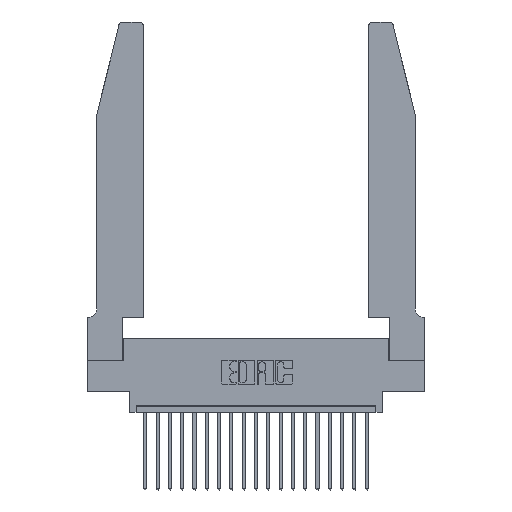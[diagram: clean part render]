
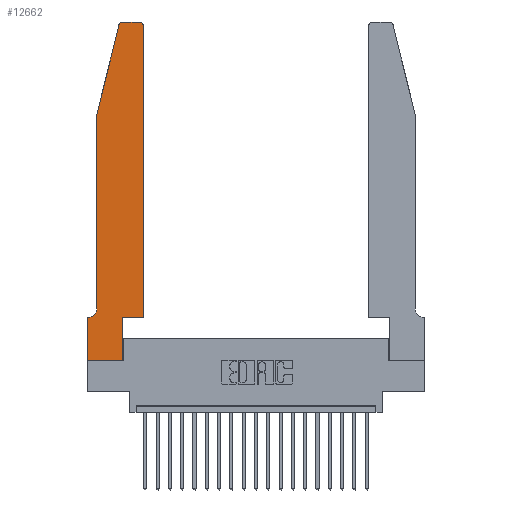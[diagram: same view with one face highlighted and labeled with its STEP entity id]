
A CAD part, top view. The second image highlights one B-rep face of the part: STEP entity #12662.
In plain terms, the highlighted planar face has unit normal (0, 0, 1).
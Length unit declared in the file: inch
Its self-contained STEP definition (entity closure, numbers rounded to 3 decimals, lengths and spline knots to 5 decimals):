
#102 = VECTOR ( 'NONE', #16913, 39.37008 ) ;
#257 = DIRECTION ( 'NONE',  ( 0., 0., -1. ) ) ;
#327 = CARTESIAN_POINT ( 'NONE',  ( 0.284, 2.75, 0.37 ) ) ;
#587 = AXIS2_PLACEMENT_3D ( 'NONE', #10549, #257, #5516 ) ;
#880 = ORIENTED_EDGE ( 'NONE', *, *, #9797, .T. ) ;
#1093 = VERTEX_POINT ( 'NONE', #22178 ) ;
#1176 = LINE ( 'NONE', #9467, #5963 ) ;
#1204 = VECTOR ( 'NONE', #10501, 39.37008 ) ;
#1364 = EDGE_CURVE ( 'NONE', #2460, #10836, #12725, .T. ) ;
#1492 = DIRECTION ( 'NONE',  ( -1., 0., 0. ) ) ;
#1579 = DIRECTION ( 'NONE',  ( 0., 0., 1. ) ) ;
#1655 = DIRECTION ( 'NONE',  ( 1., 0., 0. ) ) ;
#2086 = EDGE_LOOP ( 'NONE', ( #8079, #880, #11251, #3772, #17638, #19984, #12000, #12887, #15608, #21807, #15028, #2759 ) ) ;
#2460 = VERTEX_POINT ( 'NONE', #17323 ) ;
#2746 = LINE ( 'NONE', #17678, #9189 ) ;
#2759 = ORIENTED_EDGE ( 'NONE', *, *, #18175, .T. ) ;
#3187 = VERTEX_POINT ( 'NONE', #327 ) ;
#3426 = EDGE_CURVE ( 'NONE', #8531, #3187, #22290, .T. ) ;
#3436 = LINE ( 'NONE', #16147, #5274 ) ;
#3772 = ORIENTED_EDGE ( 'NONE', *, *, #13375, .T. ) ;
#3917 = CARTESIAN_POINT ( 'NONE',  ( 0.0755, 2., 0.37 ) ) ;
#4987 = VECTOR ( 'NONE', #1492, 39.37008 ) ;
#5092 = VECTOR ( 'NONE', #13728, 39.37008 ) ;
#5165 = LINE ( 'NONE', #13865, #1204 ) ;
#5274 = VECTOR ( 'NONE', #7617, 39.37008 ) ;
#5516 = DIRECTION ( 'NONE',  ( -1., 0., 0. ) ) ;
#5618 = CARTESIAN_POINT ( 'NONE',  ( 0.0755, 0.35, 0.37 ) ) ;
#5963 = VECTOR ( 'NONE', #7849, 39.37008 ) ;
#6348 = CARTESIAN_POINT ( 'NONE',  ( 0.4505, 0.35, 0.37 ) ) ;
#6683 = EDGE_CURVE ( 'NONE', #11929, #21466, #3436, .T. ) ;
#7617 = DIRECTION ( 'NONE',  ( 0., 1., 0. ) ) ;
#7849 = DIRECTION ( 'NONE',  ( -0.239, -0.971, 0. ) ) ;
#8027 = LINE ( 'NONE', #12352, #20471 ) ;
#8079 = ORIENTED_EDGE ( 'NONE', *, *, #3426, .T. ) ;
#8176 = CARTESIAN_POINT ( 'NONE',  ( 0.4505, 2.72, 0.37 ) ) ;
#8531 = VERTEX_POINT ( 'NONE', #11025 ) ;
#9189 = VECTOR ( 'NONE', #16290, 39.37008 ) ;
#9215 = DIRECTION ( 'NONE',  ( -1., 0., 0. ) ) ;
#9467 = CARTESIAN_POINT ( 'NONE',  ( 0.0755, 2., 0.37 ) ) ;
#9570 = EDGE_CURVE ( 'NONE', #10180, #21219, #1176, .T. ) ;
#9797 = EDGE_CURVE ( 'NONE', #3187, #10180, #21102, .T. ) ;
#9818 = CARTESIAN_POINT ( 'NONE',  ( 0.284, 2.72, 0.37 ) ) ;
#9907 = CARTESIAN_POINT ( 'NONE',  ( 0.2865, 0.35, 0.37 ) ) ;
#10023 = DIRECTION ( 'NONE',  ( 1., 0., 0. ) ) ;
#10119 = CARTESIAN_POINT ( 'NONE',  ( 0., 0.35, 0.37 ) ) ;
#10157 = VECTOR ( 'NONE', #9215, 39.37008 ) ;
#10180 = VERTEX_POINT ( 'NONE', #12488 ) ;
#10501 = DIRECTION ( 'NONE',  ( 0., -1., 0. ) ) ;
#10549 = CARTESIAN_POINT ( 'NONE',  ( 0.0055, 0.42, 0.37 ) ) ;
#10703 = EDGE_CURVE ( 'NONE', #12597, #15881, #11671, .T. ) ;
#10836 = VERTEX_POINT ( 'NONE', #12690 ) ;
#10906 = VERTEX_POINT ( 'NONE', #9907 ) ;
#11025 = CARTESIAN_POINT ( 'NONE',  ( 0.4205, 2.75, 0.37 ) ) ;
#11251 = ORIENTED_EDGE ( 'NONE', *, *, #9570, .T. ) ;
#11536 = LINE ( 'NONE', #5618, #10157 ) ;
#11671 = CIRCLE ( 'NONE', #587, 0.07 ) ;
#11929 = VERTEX_POINT ( 'NONE', #12266 ) ;
#11979 = PLANE ( 'NONE',  #20167 ) ;
#12000 = ORIENTED_EDGE ( 'NONE', *, *, #15579, .T. ) ;
#12266 = CARTESIAN_POINT ( 'NONE',  ( 0.4505, 0.35, 0.37 ) ) ;
#12352 = CARTESIAN_POINT ( 'NONE',  ( 0., 0., 0.37 ) ) ;
#12488 = CARTESIAN_POINT ( 'NONE',  ( 0.25487, 2.72718, 0.37 ) ) ;
#12597 = VERTEX_POINT ( 'NONE', #18252 ) ;
#12662 = ADVANCED_FACE ( 'NONE', ( #21810 ), #11979, .T. ) ;
#12690 = CARTESIAN_POINT ( 'NONE',  ( 0.2865, 0., 0.37 ) ) ;
#12725 = LINE ( 'NONE', #22132, #5092 ) ;
#12872 = CIRCLE ( 'NONE', #14755, 0.03 ) ;
#12887 = ORIENTED_EDGE ( 'NONE', *, *, #1364, .T. ) ;
#13375 = EDGE_CURVE ( 'NONE', #21219, #12597, #5165, .T. ) ;
#13404 = EDGE_CURVE ( 'NONE', #10906, #11929, #14656, .T. ) ;
#13728 = DIRECTION ( 'NONE',  ( 1., 0., 0. ) ) ;
#13865 = CARTESIAN_POINT ( 'NONE',  ( 0.0755, 2., 0.37 ) ) ;
#14656 = LINE ( 'NONE', #6348, #102 ) ;
#14755 = AXIS2_PLACEMENT_3D ( 'NONE', #18395, #22085, #10023 ) ;
#14777 = EDGE_CURVE ( 'NONE', #10836, #10906, #2746, .T. ) ;
#15028 = ORIENTED_EDGE ( 'NONE', *, *, #6683, .T. ) ;
#15579 = EDGE_CURVE ( 'NONE', #1093, #2460, #8027, .T. ) ;
#15608 = ORIENTED_EDGE ( 'NONE', *, *, #14777, .T. ) ;
#15784 = DIRECTION ( 'NONE',  ( 0., -1., 0. ) ) ;
#15881 = VERTEX_POINT ( 'NONE', #17670 ) ;
#16147 = CARTESIAN_POINT ( 'NONE',  ( 0.4505, 0.35, 0.37 ) ) ;
#16290 = DIRECTION ( 'NONE',  ( 0., 1., 0. ) ) ;
#16913 = DIRECTION ( 'NONE',  ( 1., 0., 0. ) ) ;
#17323 = CARTESIAN_POINT ( 'NONE',  ( 0., 0., 0.37 ) ) ;
#17638 = ORIENTED_EDGE ( 'NONE', *, *, #10703, .T. ) ;
#17670 = CARTESIAN_POINT ( 'NONE',  ( 0.0055, 0.35, 0.37 ) ) ;
#17678 = CARTESIAN_POINT ( 'NONE',  ( 0.2865, 0.35, 0.37 ) ) ;
#17866 = EDGE_CURVE ( 'NONE', #15881, #1093, #11536, .T. ) ;
#18175 = EDGE_CURVE ( 'NONE', #21466, #8531, #12872, .T. ) ;
#18252 = CARTESIAN_POINT ( 'NONE',  ( 0.0755, 0.42, 0.37 ) ) ;
#18395 = CARTESIAN_POINT ( 'NONE',  ( 0.4205, 2.72, 0.37 ) ) ;
#19984 = ORIENTED_EDGE ( 'NONE', *, *, #17866, .T. ) ;
#20167 = AXIS2_PLACEMENT_3D ( 'NONE', #10119, #1579, #1655 ) ;
#20438 = CARTESIAN_POINT ( 'NONE',  ( 0.2605, 2.75, 0.37 ) ) ;
#20471 = VECTOR ( 'NONE', #15784, 39.37008 ) ;
#20517 = DIRECTION ( 'NONE',  ( 1., 0., 0. ) ) ;
#21102 = CIRCLE ( 'NONE', #21491, 0.03 ) ;
#21219 = VERTEX_POINT ( 'NONE', #3917 ) ;
#21466 = VERTEX_POINT ( 'NONE', #8176 ) ;
#21491 = AXIS2_PLACEMENT_3D ( 'NONE', #9818, #21879, #20517 ) ;
#21807 = ORIENTED_EDGE ( 'NONE', *, *, #13404, .T. ) ;
#21810 = FACE_OUTER_BOUND ( 'NONE', #2086, .T. ) ;
#21879 = DIRECTION ( 'NONE',  ( 0., 0., 1. ) ) ;
#22085 = DIRECTION ( 'NONE',  ( 0., 0., 1. ) ) ;
#22132 = CARTESIAN_POINT ( 'NONE',  ( 0., 0., 0.37 ) ) ;
#22178 = CARTESIAN_POINT ( 'NONE',  ( 0., 0.35, 0.37 ) ) ;
#22290 = LINE ( 'NONE', #20438, #4987 ) ;
